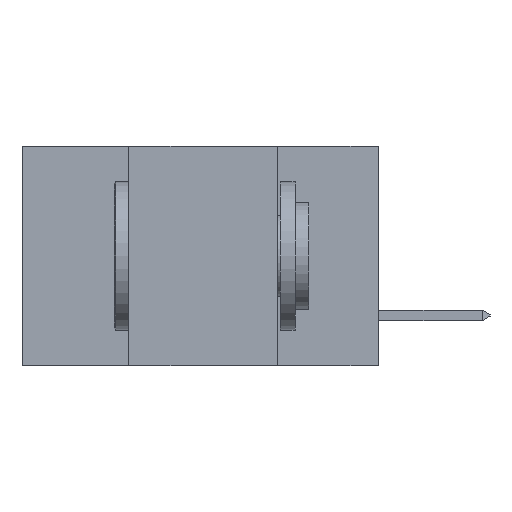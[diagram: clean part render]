
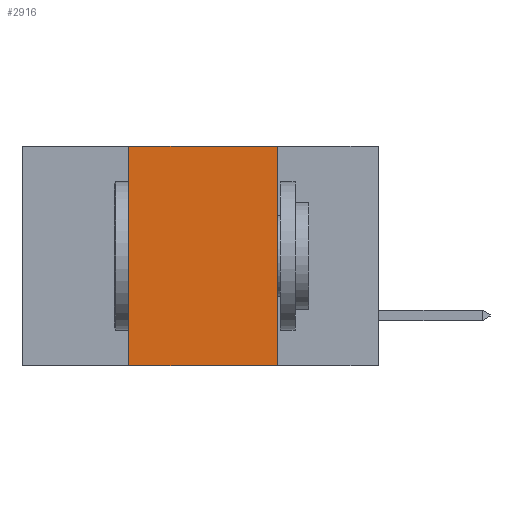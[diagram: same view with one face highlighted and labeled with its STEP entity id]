
A CAD part, left-side view. The second image highlights one B-rep face of the part: STEP entity #2916.
In plain terms, the highlighted planar face has unit normal (-1, 0, 0).
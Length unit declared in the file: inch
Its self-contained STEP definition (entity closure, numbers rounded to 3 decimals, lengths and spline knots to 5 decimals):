
#53 = CARTESIAN_POINT ( 'NONE',  ( 0., 0.6, 0. ) ) ;
#517 = ORIENTED_EDGE ( 'NONE', *, *, #1039, .F. ) ;
#998 = VERTEX_POINT ( 'NONE', #7606 ) ;
#1039 = EDGE_CURVE ( 'NONE', #6283, #998, #3781, .T. ) ;
#1171 = CARTESIAN_POINT ( 'NONE',  ( 0., 0.6, 0. ) ) ;
#1800 = LINE ( 'NONE', #6763, #7510 ) ;
#1804 = CARTESIAN_POINT ( 'NONE',  ( 0., 0.17, -0.37 ) ) ;
#2465 = VECTOR ( 'NONE', #6324, 39.37008 ) ;
#2821 = CARTESIAN_POINT ( 'NONE',  ( 0., 0.42, 0. ) ) ;
#2916 = ADVANCED_FACE ( 'NONE', ( #4305 ), #7974, .F. ) ;
#3143 = DIRECTION ( 'NONE',  ( 0., 0., -1. ) ) ;
#3452 = DIRECTION ( 'NONE',  ( 0., -1., 0. ) ) ;
#3494 = CARTESIAN_POINT ( 'NONE',  ( 0., 0.6, -0.37 ) ) ;
#3565 = VECTOR ( 'NONE', #3452, 39.37008 ) ;
#3781 = LINE ( 'NONE', #53, #3565 ) ;
#3804 = DIRECTION ( 'NONE',  ( 1., 0., 0. ) ) ;
#3898 = CARTESIAN_POINT ( 'NONE',  ( 0., 0.42, -0.37 ) ) ;
#3987 = AXIS2_PLACEMENT_3D ( 'NONE', #1171, #3804, #3143 ) ;
#4083 = LINE ( 'NONE', #1804, #5963 ) ;
#4305 = FACE_OUTER_BOUND ( 'NONE', #6262, .T. ) ;
#4412 = ORIENTED_EDGE ( 'NONE', *, *, #5631, .F. ) ;
#5527 = VERTEX_POINT ( 'NONE', #7702 ) ;
#5631 = EDGE_CURVE ( 'NONE', #6039, #6283, #1800, .T. ) ;
#5963 = VECTOR ( 'NONE', #6141, 39.37008 ) ;
#6039 = VERTEX_POINT ( 'NONE', #3898 ) ;
#6089 = ORIENTED_EDGE ( 'NONE', *, *, #8631, .F. ) ;
#6141 = DIRECTION ( 'NONE',  ( 0., 0., -1. ) ) ;
#6262 = EDGE_LOOP ( 'NONE', ( #6089, #517, #4412, #8338 ) ) ;
#6283 = VERTEX_POINT ( 'NONE', #2821 ) ;
#6324 = DIRECTION ( 'NONE',  ( 0., -1., 0. ) ) ;
#6673 = DIRECTION ( 'NONE',  ( 0., 0., 1. ) ) ;
#6763 = CARTESIAN_POINT ( 'NONE',  ( 0., 0.42, -0.37 ) ) ;
#7057 = EDGE_CURVE ( 'NONE', #6039, #5527, #8135, .T. ) ;
#7510 = VECTOR ( 'NONE', #6673, 39.37008 ) ;
#7606 = CARTESIAN_POINT ( 'NONE',  ( 0., 0.17, 0. ) ) ;
#7702 = CARTESIAN_POINT ( 'NONE',  ( 0., 0.17, -0.37 ) ) ;
#7974 = PLANE ( 'NONE',  #3987 ) ;
#8135 = LINE ( 'NONE', #3494, #2465 ) ;
#8338 = ORIENTED_EDGE ( 'NONE', *, *, #7057, .T. ) ;
#8631 = EDGE_CURVE ( 'NONE', #998, #5527, #4083, .T. ) ;
